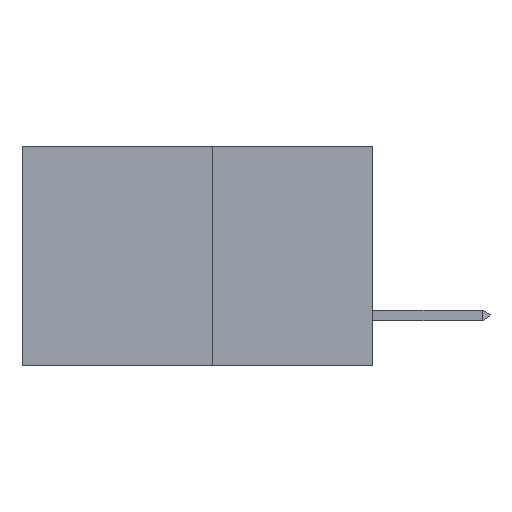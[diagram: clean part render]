
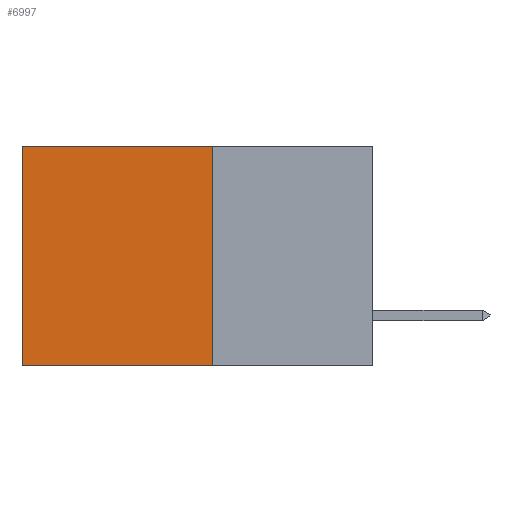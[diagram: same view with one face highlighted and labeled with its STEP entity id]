
A CAD part, left-side view. The second image highlights one B-rep face of the part: STEP entity #6997.
In plain terms, the highlighted planar face has unit normal (-1, 0, 0).
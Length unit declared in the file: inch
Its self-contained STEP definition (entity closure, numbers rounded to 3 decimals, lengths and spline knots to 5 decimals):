
#244 = ORIENTED_EDGE ( 'NONE', *, *, #19113, .F. ) ;
#1322 = LINE ( 'NONE', #10124, #24721 ) ;
#2921 = VERTEX_POINT ( 'NONE', #14875 ) ;
#5903 = ORIENTED_EDGE ( 'NONE', *, *, #17839, .F. ) ;
#6658 = VERTEX_POINT ( 'NONE', #9249 ) ;
#6997 = ADVANCED_FACE ( 'NONE', ( #23578 ), #29723, .F. ) ;
#7106 = EDGE_LOOP ( 'NONE', ( #8458, #244, #5903, #12782 ) ) ;
#8458 = ORIENTED_EDGE ( 'NONE', *, *, #13913, .T. ) ;
#9249 = CARTESIAN_POINT ( 'NONE',  ( 0.277, 0.27, 0. ) ) ;
#9946 = VECTOR ( 'NONE', #21562, 39.37008 ) ;
#9960 = CARTESIAN_POINT ( 'NONE',  ( 0.277, 0.59, -0.37 ) ) ;
#10124 = CARTESIAN_POINT ( 'NONE',  ( 0.277, 0.27, -0.37 ) ) ;
#10673 = LINE ( 'NONE', #9960, #9946 ) ;
#11786 = LINE ( 'NONE', #27544, #24870 ) ;
#12676 = CARTESIAN_POINT ( 'NONE',  ( 0.277, 0.59, 0. ) ) ;
#12782 = ORIENTED_EDGE ( 'NONE', *, *, #13605, .T. ) ;
#13486 = LINE ( 'NONE', #24413, #25122 ) ;
#13605 = EDGE_CURVE ( 'NONE', #6658, #28814, #11786, .T. ) ;
#13629 = DIRECTION ( 'NONE',  ( 0., 1., 0. ) ) ;
#13913 = EDGE_CURVE ( 'NONE', #28814, #26411, #10673, .T. ) ;
#14875 = CARTESIAN_POINT ( 'NONE',  ( 0.277, 0.27, -0.37 ) ) ;
#15226 = AXIS2_PLACEMENT_3D ( 'NONE', #29380, #29129, #29093 ) ;
#17839 = EDGE_CURVE ( 'NONE', #6658, #2921, #13486, .T. ) ;
#18429 = CARTESIAN_POINT ( 'NONE',  ( 0.277, 0.59, -0.37 ) ) ;
#19113 = EDGE_CURVE ( 'NONE', #2921, #26411, #1322, .T. ) ;
#21562 = DIRECTION ( 'NONE',  ( 0., 0., -1. ) ) ;
#23578 = FACE_OUTER_BOUND ( 'NONE', #7106, .T. ) ;
#24413 = CARTESIAN_POINT ( 'NONE',  ( 0.277, 0.27, -0.37 ) ) ;
#24721 = VECTOR ( 'NONE', #28694, 39.37008 ) ;
#24870 = VECTOR ( 'NONE', #13629, 39.37008 ) ;
#25122 = VECTOR ( 'NONE', #26762, 39.37008 ) ;
#26411 = VERTEX_POINT ( 'NONE', #18429 ) ;
#26762 = DIRECTION ( 'NONE',  ( 0., 0., -1. ) ) ;
#27544 = CARTESIAN_POINT ( 'NONE',  ( 0.277, 0.27, 0. ) ) ;
#28694 = DIRECTION ( 'NONE',  ( 0., 1., 0. ) ) ;
#28814 = VERTEX_POINT ( 'NONE', #12676 ) ;
#29093 = DIRECTION ( 'NONE',  ( 0., 0., -1. ) ) ;
#29129 = DIRECTION ( 'NONE',  ( 1., 0., 0. ) ) ;
#29380 = CARTESIAN_POINT ( 'NONE',  ( 0.277, 0.27, -0.37 ) ) ;
#29723 = PLANE ( 'NONE',  #15226 ) ;
